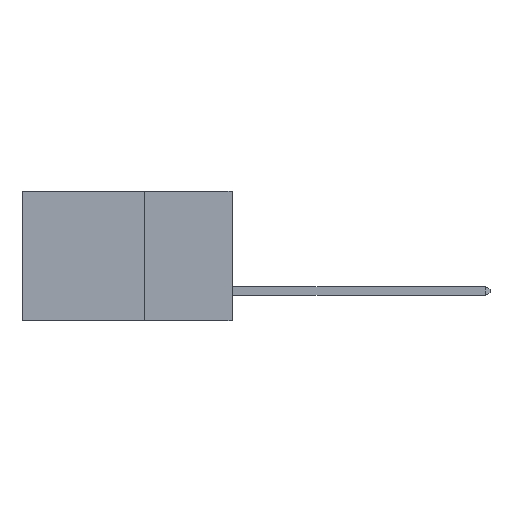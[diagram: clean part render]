
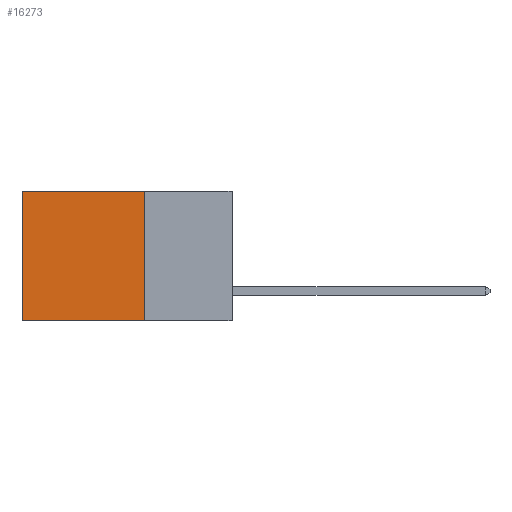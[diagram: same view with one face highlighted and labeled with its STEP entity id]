
A CAD part, left-side view. The second image highlights one B-rep face of the part: STEP entity #16273.
In plain terms, the highlighted planar face has unit normal (-1, 0, 0).
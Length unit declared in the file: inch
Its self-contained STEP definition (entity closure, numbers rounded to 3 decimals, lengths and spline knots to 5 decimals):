
#227 = DIRECTION ( 'NONE',  ( 0., 0., -1. ) ) ;
#513 = VECTOR ( 'NONE', #13393, 39.37008 ) ;
#2010 = DIRECTION ( 'NONE',  ( 0., 0., -1. ) ) ;
#2787 = EDGE_CURVE ( 'NONE', #18760, #20463, #16823, .T. ) ;
#2839 = CARTESIAN_POINT ( 'NONE',  ( 0.2875, 0.25, 0. ) ) ;
#3302 = CARTESIAN_POINT ( 'NONE',  ( 0.2875, 0.25, 0. ) ) ;
#3452 = VECTOR ( 'NONE', #18266, 39.37008 ) ;
#3991 = LINE ( 'NONE', #4941, #3452 ) ;
#4906 = CARTESIAN_POINT ( 'NONE',  ( 0.2875, 0.25, -0.37 ) ) ;
#4941 = CARTESIAN_POINT ( 'NONE',  ( 0.2875, 0.25, -0.37 ) ) ;
#4969 = LINE ( 'NONE', #20407, #17233 ) ;
#5125 = LINE ( 'NONE', #3302, #513 ) ;
#5740 = EDGE_CURVE ( 'NONE', #20463, #6011, #4969, .T. ) ;
#6011 = VERTEX_POINT ( 'NONE', #16167 ) ;
#6235 = AXIS2_PLACEMENT_3D ( 'NONE', #7085, #10477, #227 ) ;
#7085 = CARTESIAN_POINT ( 'NONE',  ( 0.2875, 0.25, 0. ) ) ;
#7336 = EDGE_CURVE ( 'NONE', #16711, #6011, #3991, .T. ) ;
#10344 = ORIENTED_EDGE ( 'NONE', *, *, #7336, .F. ) ;
#10477 = DIRECTION ( 'NONE',  ( 1., 0., 0. ) ) ;
#10505 = ORIENTED_EDGE ( 'NONE', *, *, #2787, .T. ) ;
#11256 = FACE_OUTER_BOUND ( 'NONE', #20308, .T. ) ;
#12330 = EDGE_CURVE ( 'NONE', #18760, #16711, #5125, .T. ) ;
#13393 = DIRECTION ( 'NONE',  ( 0., 0., -1. ) ) ;
#16167 = CARTESIAN_POINT ( 'NONE',  ( 0.2875, 0.6, -0.37 ) ) ;
#16273 = ADVANCED_FACE ( 'NONE', ( #11256 ), #20327, .F. ) ;
#16711 = VERTEX_POINT ( 'NONE', #4906 ) ;
#16823 = LINE ( 'NONE', #2839, #20648 ) ;
#17233 = VECTOR ( 'NONE', #2010, 39.37008 ) ;
#18266 = DIRECTION ( 'NONE',  ( 0., 1., 0. ) ) ;
#18760 = VERTEX_POINT ( 'NONE', #19828 ) ;
#18905 = ORIENTED_EDGE ( 'NONE', *, *, #5740, .T. ) ;
#19828 = CARTESIAN_POINT ( 'NONE',  ( 0.2875, 0.25, 0. ) ) ;
#20308 = EDGE_LOOP ( 'NONE', ( #18905, #10344, #20731, #10505 ) ) ;
#20327 = PLANE ( 'NONE',  #6235 ) ;
#20407 = CARTESIAN_POINT ( 'NONE',  ( 0.2875, 0.6, 0. ) ) ;
#20463 = VERTEX_POINT ( 'NONE', #20989 ) ;
#20648 = VECTOR ( 'NONE', #21214, 39.37008 ) ;
#20731 = ORIENTED_EDGE ( 'NONE', *, *, #12330, .F. ) ;
#20989 = CARTESIAN_POINT ( 'NONE',  ( 0.2875, 0.6, 0. ) ) ;
#21214 = DIRECTION ( 'NONE',  ( 0., 1., 0. ) ) ;
